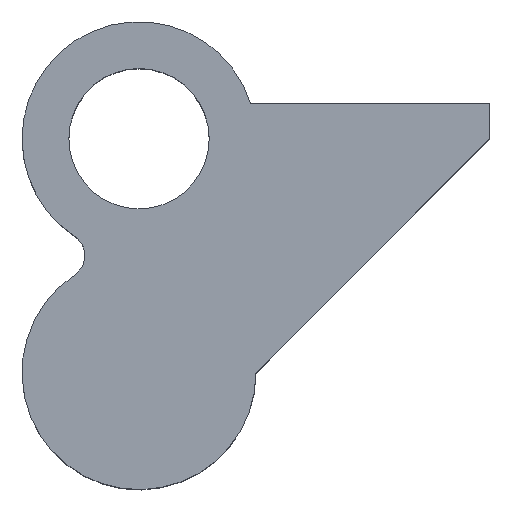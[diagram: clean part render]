
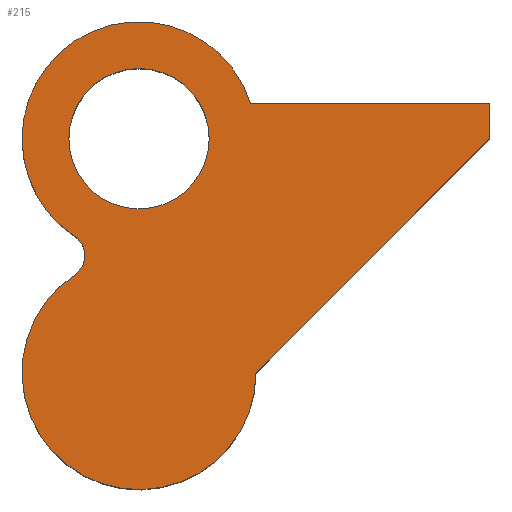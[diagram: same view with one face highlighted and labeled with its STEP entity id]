
A CAD part, top view. The second image highlights one B-rep face of the part: STEP entity #215.
In plain terms, the highlighted planar face has unit normal (0, 0, 1).
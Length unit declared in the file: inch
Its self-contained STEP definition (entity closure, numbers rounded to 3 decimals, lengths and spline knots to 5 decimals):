
#4 = DIRECTION ( 'NONE',  ( 0., 0., 1. ) ) ;
#6 = CARTESIAN_POINT ( 'NONE',  ( -3.03213, 0., 0.3937 ) ) ;
#18 = ORIENTED_EDGE ( 'NONE', *, *, #368, .F. ) ;
#20 = LINE ( 'NONE', #120, #158 ) ;
#29 = CIRCLE ( 'NONE', #295, 0.03937 ) ;
#33 = ORIENTED_EDGE ( 'NONE', *, *, #365, .T. ) ;
#34 = DIRECTION ( 'NONE',  ( 0., 0., 1. ) ) ;
#48 = CARTESIAN_POINT ( 'NONE',  ( -3.7315, -1.47966, 0.3937 ) ) ;
#51 = VERTEX_POINT ( 'NONE', #152 ) ;
#54 = EDGE_LOOP ( 'NONE', ( #333, #177, #33, #147, #18, #281, #292 ) ) ;
#58 = CARTESIAN_POINT ( 'NONE',  ( -3.62268, -1.25, 0.3937 ) ) ;
#64 = ORIENTED_EDGE ( 'NONE', *, *, #350, .F. ) ;
#84 = DIRECTION ( 'NONE',  ( 1., 0., 0. ) ) ;
#89 = DIRECTION ( 'NONE',  ( 1., 0., 0. ) ) ;
#96 = VECTOR ( 'NONE', #117, 39.37008 ) ;
#98 = DIRECTION ( 'NONE',  ( 0., 0., 1. ) ) ;
#104 = CIRCLE ( 'NONE', #296, 0.19685 ) ;
#105 = VERTEX_POINT ( 'NONE', #249 ) ;
#109 = FACE_OUTER_BOUND ( 'NONE', #54, .T. ) ;
#113 = LINE ( 'NONE', #6, #305 ) ;
#117 = DIRECTION ( 'NONE',  ( -0.707, -0.707, 0. ) ) ;
#120 = CARTESIAN_POINT ( 'NONE',  ( -3.03213, -1.19094, 0.3937 ) ) ;
#126 = CIRCLE ( 'NONE', #315, 0.11811 ) ;
#127 = VERTEX_POINT ( 'NONE', #228 ) ;
#142 = DIRECTION ( 'NONE',  ( 0., 0., -1. ) ) ;
#144 = DIRECTION ( 'NONE',  ( 1., 0., 0. ) ) ;
#147 = ORIENTED_EDGE ( 'NONE', *, *, #367, .T. ) ;
#151 = VERTEX_POINT ( 'NONE', #334 ) ;
#152 = CARTESIAN_POINT ( 'NONE',  ( -3.81953, -1.25, 0.3937 ) ) ;
#157 = CARTESIAN_POINT ( 'NONE',  ( -3.42583, -1.6437, 0.3937 ) ) ;
#158 = VECTOR ( 'NONE', #144, 39.37008 ) ;
#165 = DIRECTION ( 'NONE',  ( 0., 0., 1. ) ) ;
#171 = CARTESIAN_POINT ( 'NONE',  ( -3.62268, -1.25, 0.3937 ) ) ;
#177 = ORIENTED_EDGE ( 'NONE', *, *, #348, .T. ) ;
#184 = DIRECTION ( 'NONE',  ( 1., 0., 0. ) ) ;
#192 = DIRECTION ( 'NONE',  ( 1., 0., 0. ) ) ;
#195 = CARTESIAN_POINT ( 'NONE',  ( -3.62268, -1.6437, 0.3937 ) ) ;
#207 = VERTEX_POINT ( 'NONE', #48 ) ;
#212 = CARTESIAN_POINT ( 'NONE',  ( -3.62268, -1.25, 0.3937 ) ) ;
#215 = ADVANCED_FACE ( 'NONE', ( #233, #109 ), #294, .T. ) ;
#217 = DIRECTION ( 'NONE',  ( 1., 0., 0. ) ) ;
#221 = VERTEX_POINT ( 'NONE', #157 ) ;
#228 = CARTESIAN_POINT ( 'NONE',  ( -3.74079, -1.25, 0.3937 ) ) ;
#230 = LINE ( 'NONE', #269, #96 ) ;
#233 = FACE_BOUND ( 'NONE', #377, .T. ) ;
#234 = AXIS2_PLACEMENT_3D ( 'NONE', #336, #378, #184 ) ;
#237 = CIRCLE ( 'NONE', #300, 0.11811 ) ;
#241 = DIRECTION ( 'NONE',  ( 0., 0., 1. ) ) ;
#242 = DIRECTION ( 'NONE',  ( 0., 1., 0. ) ) ;
#245 = VERTEX_POINT ( 'NONE', #337 ) ;
#249 = CARTESIAN_POINT ( 'NONE',  ( -3.03213, -1.19094, 0.3937 ) ) ;
#253 = VERTEX_POINT ( 'NONE', #381 ) ;
#265 = CIRCLE ( 'NONE', #323, 0.19685 ) ;
#269 = CARTESIAN_POINT ( 'NONE',  ( -0.89107, 0.89107, 0.3937 ) ) ;
#276 = ORIENTED_EDGE ( 'NONE', *, *, #359, .F. ) ;
#277 = CARTESIAN_POINT ( 'NONE',  ( -3.50457, -1.25, 0.3937 ) ) ;
#281 = ORIENTED_EDGE ( 'NONE', *, *, #369, .T. ) ;
#291 = AXIS2_PLACEMENT_3D ( 'NONE', #195, #34, #217 ) ;
#292 = ORIENTED_EDGE ( 'NONE', *, *, #370, .F. ) ;
#294 = PLANE ( 'NONE',  #234 ) ;
#295 = AXIS2_PLACEMENT_3D ( 'NONE', #310, #142, #352 ) ;
#296 = AXIS2_PLACEMENT_3D ( 'NONE', #58, #241, #89 ) ;
#300 = AXIS2_PLACEMENT_3D ( 'NONE', #171, #4, #192 ) ;
#305 = VECTOR ( 'NONE', #242, 39.37008 ) ;
#310 = CARTESIAN_POINT ( 'NONE',  ( -3.75326, -1.44685, 0.3937 ) ) ;
#315 = AXIS2_PLACEMENT_3D ( 'NONE', #212, #98, #84 ) ;
#321 = CIRCLE ( 'NONE', #291, 0.19685 ) ;
#323 = AXIS2_PLACEMENT_3D ( 'NONE', #343, #165, #385 ) ;
#333 = ORIENTED_EDGE ( 'NONE', *, *, #362, .T. ) ;
#334 = CARTESIAN_POINT ( 'NONE',  ( -3.4349, -1.19094, 0.3937 ) ) ;
#336 = CARTESIAN_POINT ( 'NONE',  ( 0., 0., 0.3937 ) ) ;
#337 = CARTESIAN_POINT ( 'NONE',  ( -3.7315, -1.41404, 0.3937 ) ) ;
#343 = CARTESIAN_POINT ( 'NONE',  ( -3.62268, -1.25, 0.3937 ) ) ;
#348 = EDGE_CURVE ( 'NONE', #51, #245, #265, .T. ) ;
#350 = EDGE_CURVE ( 'NONE', #127, #391, #126, .T. ) ;
#352 = DIRECTION ( 'NONE',  ( 1., 0., 0. ) ) ;
#359 = EDGE_CURVE ( 'NONE', #391, #127, #237, .T. ) ;
#362 = EDGE_CURVE ( 'NONE', #151, #51, #104, .T. ) ;
#365 = EDGE_CURVE ( 'NONE', #245, #207, #29, .T. ) ;
#367 = EDGE_CURVE ( 'NONE', #207, #221, #321, .T. ) ;
#368 = EDGE_CURVE ( 'NONE', #253, #221, #230, .T. ) ;
#369 = EDGE_CURVE ( 'NONE', #253, #105, #113, .T. ) ;
#370 = EDGE_CURVE ( 'NONE', #151, #105, #20, .T. ) ;
#377 = EDGE_LOOP ( 'NONE', ( #64, #276 ) ) ;
#378 = DIRECTION ( 'NONE',  ( 0., 0., 1. ) ) ;
#381 = CARTESIAN_POINT ( 'NONE',  ( -3.03213, -1.25, 0.3937 ) ) ;
#385 = DIRECTION ( 'NONE',  ( 1., 0., 0. ) ) ;
#391 = VERTEX_POINT ( 'NONE', #277 ) ;
